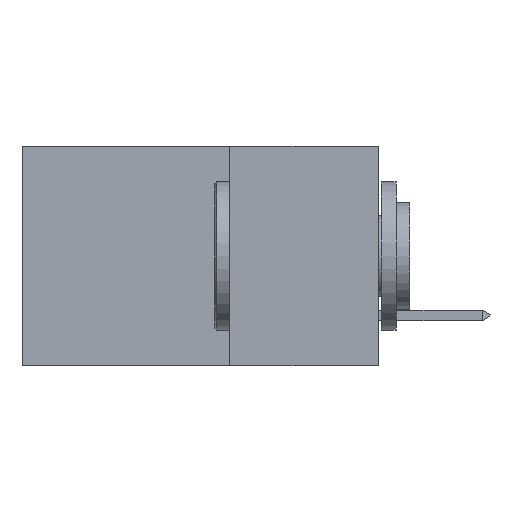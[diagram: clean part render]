
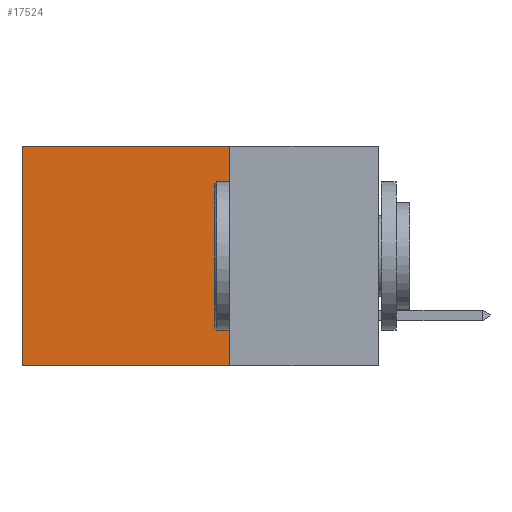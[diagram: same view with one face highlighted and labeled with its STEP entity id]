
A CAD part, left-side view. The second image highlights one B-rep face of the part: STEP entity #17524.
In plain terms, the highlighted planar face has unit normal (-1, 0, 0).
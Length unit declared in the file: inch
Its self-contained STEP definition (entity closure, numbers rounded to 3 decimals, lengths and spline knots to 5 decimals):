
#2050 = CARTESIAN_POINT ( 'NONE',  ( 0.2615, 0.25, -0.37 ) ) ;
#3168 = PLANE ( 'NONE',  #10743 ) ;
#3258 = LINE ( 'NONE', #6566, #7323 ) ;
#3281 = FACE_OUTER_BOUND ( 'NONE', #12648, .T. ) ;
#3368 = DIRECTION ( 'NONE',  ( 0., 1., 0. ) ) ;
#3428 = CARTESIAN_POINT ( 'NONE',  ( 0.2615, 0.25, 0. ) ) ;
#3628 = CARTESIAN_POINT ( 'NONE',  ( 0.2615, 0.25, -0.37 ) ) ;
#3700 = EDGE_CURVE ( 'NONE', #5643, #8414, #17063, .T. ) ;
#4948 = ORIENTED_EDGE ( 'NONE', *, *, #17996, .F. ) ;
#5375 = VECTOR ( 'NONE', #20467, 39.37008 ) ;
#5387 = EDGE_CURVE ( 'NONE', #7617, #18567, #6626, .T. ) ;
#5636 = CARTESIAN_POINT ( 'NONE',  ( 0.2615, 0.6, -0.37 ) ) ;
#5643 = VERTEX_POINT ( 'NONE', #16056 ) ;
#6385 = VECTOR ( 'NONE', #11988, 39.37008 ) ;
#6566 = CARTESIAN_POINT ( 'NONE',  ( 0.2615, 0.25, -0.37 ) ) ;
#6626 = LINE ( 'NONE', #3628, #6385 ) ;
#7323 = VECTOR ( 'NONE', #3368, 39.37008 ) ;
#7617 = VERTEX_POINT ( 'NONE', #13883 ) ;
#7785 = EDGE_CURVE ( 'NONE', #7617, #5643, #8253, .T. ) ;
#8067 = ORIENTED_EDGE ( 'NONE', *, *, #7785, .T. ) ;
#8253 = LINE ( 'NONE', #3428, #11520 ) ;
#8414 = VERTEX_POINT ( 'NONE', #5636 ) ;
#8914 = CARTESIAN_POINT ( 'NONE',  ( 0.2615, 0.6, -0.37 ) ) ;
#9603 = DIRECTION ( 'NONE',  ( 0., 0., -1. ) ) ;
#10743 = AXIS2_PLACEMENT_3D ( 'NONE', #17943, #21159, #9603 ) ;
#11520 = VECTOR ( 'NONE', #16510, 39.37008 ) ;
#11988 = DIRECTION ( 'NONE',  ( 0., 0., -1. ) ) ;
#12612 = ORIENTED_EDGE ( 'NONE', *, *, #5387, .F. ) ;
#12648 = EDGE_LOOP ( 'NONE', ( #14732, #4948, #12612, #8067 ) ) ;
#13883 = CARTESIAN_POINT ( 'NONE',  ( 0.2615, 0.25, 0. ) ) ;
#14732 = ORIENTED_EDGE ( 'NONE', *, *, #3700, .T. ) ;
#16056 = CARTESIAN_POINT ( 'NONE',  ( 0.2615, 0.6, 0. ) ) ;
#16510 = DIRECTION ( 'NONE',  ( 0., 1., 0. ) ) ;
#17063 = LINE ( 'NONE', #8914, #5375 ) ;
#17524 = ADVANCED_FACE ( 'NONE', ( #3281 ), #3168, .F. ) ;
#17943 = CARTESIAN_POINT ( 'NONE',  ( 0.2615, 0.25, -0.37 ) ) ;
#17996 = EDGE_CURVE ( 'NONE', #18567, #8414, #3258, .T. ) ;
#18567 = VERTEX_POINT ( 'NONE', #2050 ) ;
#20467 = DIRECTION ( 'NONE',  ( 0., 0., -1. ) ) ;
#21159 = DIRECTION ( 'NONE',  ( 1., 0., 0. ) ) ;
